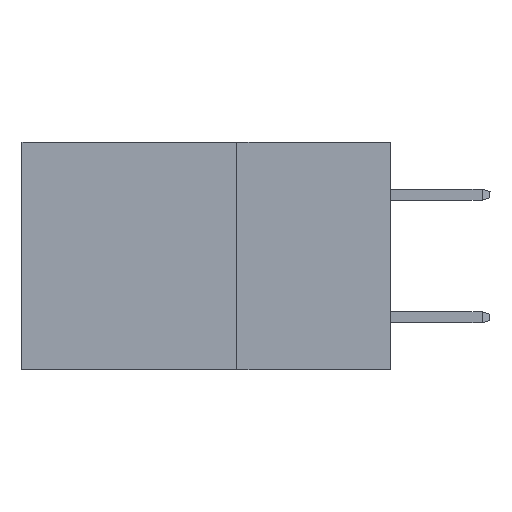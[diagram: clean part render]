
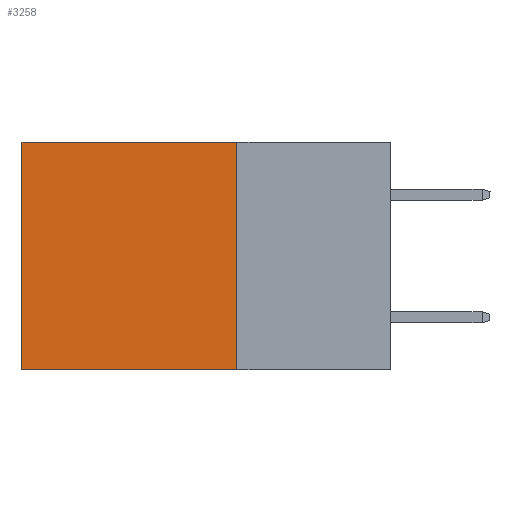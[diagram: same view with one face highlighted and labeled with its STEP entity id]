
A CAD part, left-side view. The second image highlights one B-rep face of the part: STEP entity #3258.
In plain terms, the highlighted planar face has unit normal (-1, 0, 0).
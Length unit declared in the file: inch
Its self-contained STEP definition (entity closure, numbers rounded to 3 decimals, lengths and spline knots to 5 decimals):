
#28 = VECTOR ( 'NONE', #6762, 39.37008 ) ;
#182 = CARTESIAN_POINT ( 'NONE',  ( 0.2875, 0.25, 0. ) ) ;
#295 = VECTOR ( 'NONE', #11739, 39.37008 ) ;
#817 = EDGE_LOOP ( 'NONE', ( #2100, #3915, #10406, #10197 ) ) ;
#1338 = EDGE_CURVE ( 'NONE', #9978, #4142, #14790, .T. ) ;
#1893 = VECTOR ( 'NONE', #14549, 39.37008 ) ;
#2100 = ORIENTED_EDGE ( 'NONE', *, *, #3376, .T. ) ;
#2283 = LINE ( 'NONE', #13443, #1893 ) ;
#3205 = DIRECTION ( 'NONE',  ( 0., 0., -1. ) ) ;
#3258 = ADVANCED_FACE ( 'NONE', ( #5064 ), #4584, .F. ) ;
#3376 = EDGE_CURVE ( 'NONE', #4142, #11701, #12323, .T. ) ;
#3705 = VECTOR ( 'NONE', #3205, 39.37008 ) ;
#3915 = ORIENTED_EDGE ( 'NONE', *, *, #12054, .F. ) ;
#4142 = VERTEX_POINT ( 'NONE', #9039 ) ;
#4529 = CARTESIAN_POINT ( 'NONE',  ( 0.2875, 0.25, 0. ) ) ;
#4584 = PLANE ( 'NONE',  #11362 ) ;
#5064 = FACE_OUTER_BOUND ( 'NONE', #817, .T. ) ;
#6762 = DIRECTION ( 'NONE',  ( 0., 0., -1. ) ) ;
#6978 = DIRECTION ( 'NONE',  ( 1., 0., 0. ) ) ;
#9039 = CARTESIAN_POINT ( 'NONE',  ( 0.2875, 0.6, 0. ) ) ;
#9555 = CARTESIAN_POINT ( 'NONE',  ( 0.2875, 0.25, 0. ) ) ;
#9616 = EDGE_CURVE ( 'NONE', #9978, #12845, #9750, .T. ) ;
#9750 = LINE ( 'NONE', #12254, #3705 ) ;
#9978 = VERTEX_POINT ( 'NONE', #9555 ) ;
#10197 = ORIENTED_EDGE ( 'NONE', *, *, #1338, .T. ) ;
#10406 = ORIENTED_EDGE ( 'NONE', *, *, #9616, .F. ) ;
#10636 = CARTESIAN_POINT ( 'NONE',  ( 0.2875, 0.6, -0.37 ) ) ;
#11362 = AXIS2_PLACEMENT_3D ( 'NONE', #4529, #6978, #14321 ) ;
#11626 = CARTESIAN_POINT ( 'NONE',  ( 0.2875, 0.25, -0.37 ) ) ;
#11701 = VERTEX_POINT ( 'NONE', #10636 ) ;
#11739 = DIRECTION ( 'NONE',  ( 0., 1., 0. ) ) ;
#12054 = EDGE_CURVE ( 'NONE', #12845, #11701, #2283, .T. ) ;
#12076 = CARTESIAN_POINT ( 'NONE',  ( 0.2875, 0.6, 0. ) ) ;
#12254 = CARTESIAN_POINT ( 'NONE',  ( 0.2875, 0.25, 0. ) ) ;
#12323 = LINE ( 'NONE', #12076, #28 ) ;
#12845 = VERTEX_POINT ( 'NONE', #11626 ) ;
#13443 = CARTESIAN_POINT ( 'NONE',  ( 0.2875, 0.25, -0.37 ) ) ;
#14321 = DIRECTION ( 'NONE',  ( 0., 0., -1. ) ) ;
#14549 = DIRECTION ( 'NONE',  ( 0., 1., 0. ) ) ;
#14790 = LINE ( 'NONE', #182, #295 ) ;
